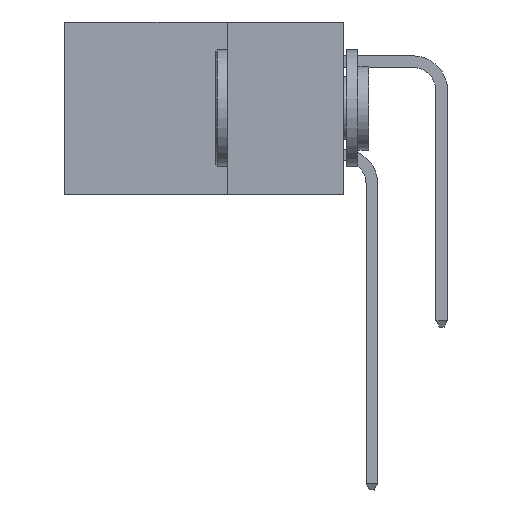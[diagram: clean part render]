
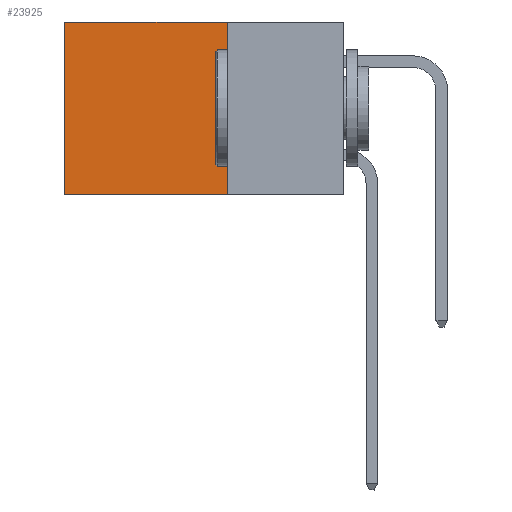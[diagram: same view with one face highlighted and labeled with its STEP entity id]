
A CAD part, left-side view. The second image highlights one B-rep face of the part: STEP entity #23925.
In plain terms, the highlighted planar face has unit normal (-1, 0, 0).
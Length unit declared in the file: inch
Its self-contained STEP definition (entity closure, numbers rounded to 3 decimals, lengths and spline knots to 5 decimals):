
#1250 = ORIENTED_EDGE ( 'NONE', *, *, #1828, .F. ) ;
#1282 = LINE ( 'NONE', #28652, #14584 ) ;
#1828 = EDGE_CURVE ( 'NONE', #4095, #30812, #3156, .T. ) ;
#3156 = LINE ( 'NONE', #16121, #18704 ) ;
#4095 = VERTEX_POINT ( 'NONE', #29798 ) ;
#6077 = EDGE_CURVE ( 'NONE', #27598, #32645, #1282, .T. ) ;
#7107 = CARTESIAN_POINT ( 'NONE',  ( 0.298, 0.25, 0. ) ) ;
#8089 = CARTESIAN_POINT ( 'NONE',  ( 0.298, 0.6, -0.37 ) ) ;
#8462 = LINE ( 'NONE', #24202, #11035 ) ;
#8706 = CARTESIAN_POINT ( 'NONE',  ( 0.298, 0.6, 0. ) ) ;
#9182 = DIRECTION ( 'NONE',  ( 0., 1., 0. ) ) ;
#11035 = VECTOR ( 'NONE', #16271, 39.37008 ) ;
#12538 = EDGE_CURVE ( 'NONE', #27598, #4095, #8462, .T. ) ;
#13430 = ORIENTED_EDGE ( 'NONE', *, *, #12538, .F. ) ;
#14584 = VECTOR ( 'NONE', #9182, 39.37008 ) ;
#15695 = CARTESIAN_POINT ( 'NONE',  ( 0.298, 0.6, 0. ) ) ;
#16121 = CARTESIAN_POINT ( 'NONE',  ( 0.298, 0.25, -0.37 ) ) ;
#16271 = DIRECTION ( 'NONE',  ( 0., 0., -1. ) ) ;
#18057 = AXIS2_PLACEMENT_3D ( 'NONE', #24828, #27254, #24945 ) ;
#18517 = ORIENTED_EDGE ( 'NONE', *, *, #6077, .T. ) ;
#18704 = VECTOR ( 'NONE', #18936, 39.37008 ) ;
#18936 = DIRECTION ( 'NONE',  ( 0., 1., 0. ) ) ;
#19042 = VECTOR ( 'NONE', #21161, 39.37008 ) ;
#19424 = EDGE_CURVE ( 'NONE', #32645, #30812, #34934, .T. ) ;
#21161 = DIRECTION ( 'NONE',  ( 0., 0., -1. ) ) ;
#21658 = EDGE_LOOP ( 'NONE', ( #22120, #1250, #13430, #18517 ) ) ;
#21662 = FACE_OUTER_BOUND ( 'NONE', #21658, .T. ) ;
#22068 = PLANE ( 'NONE',  #18057 ) ;
#22120 = ORIENTED_EDGE ( 'NONE', *, *, #19424, .T. ) ;
#23925 = ADVANCED_FACE ( 'NONE', ( #21662 ), #22068, .F. ) ;
#24202 = CARTESIAN_POINT ( 'NONE',  ( 0.298, 0.25, 0. ) ) ;
#24828 = CARTESIAN_POINT ( 'NONE',  ( 0.298, 0.25, 0. ) ) ;
#24945 = DIRECTION ( 'NONE',  ( 0., 0., -1. ) ) ;
#27254 = DIRECTION ( 'NONE',  ( 1., 0., 0. ) ) ;
#27598 = VERTEX_POINT ( 'NONE', #7107 ) ;
#28652 = CARTESIAN_POINT ( 'NONE',  ( 0.298, 0.25, 0. ) ) ;
#29798 = CARTESIAN_POINT ( 'NONE',  ( 0.298, 0.25, -0.37 ) ) ;
#30812 = VERTEX_POINT ( 'NONE', #8089 ) ;
#32645 = VERTEX_POINT ( 'NONE', #8706 ) ;
#34934 = LINE ( 'NONE', #15695, #19042 ) ;
